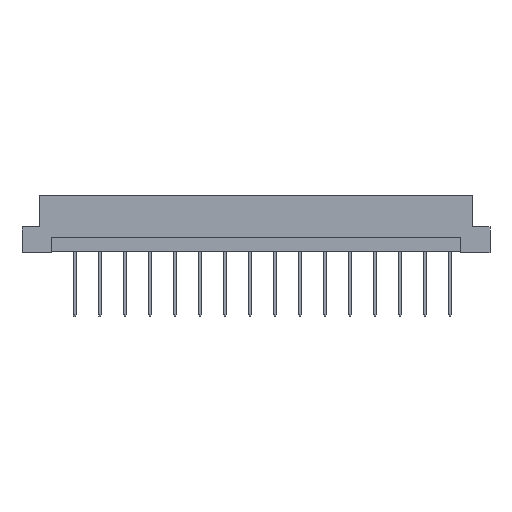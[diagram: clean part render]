
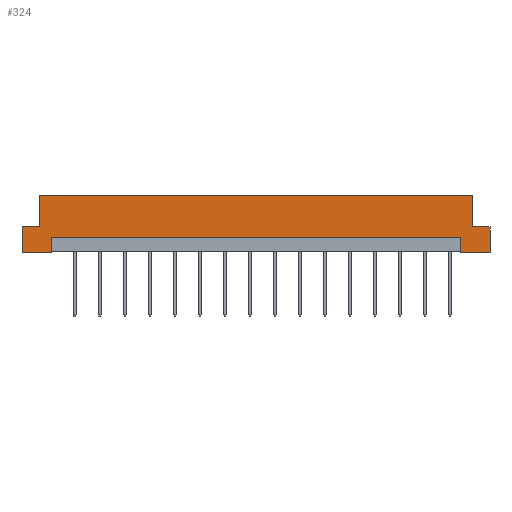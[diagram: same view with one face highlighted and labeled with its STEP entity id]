
A CAD part, front view. The second image highlights one B-rep face of the part: STEP entity #324.
In plain terms, the highlighted planar face has unit normal (0, -1, 0).
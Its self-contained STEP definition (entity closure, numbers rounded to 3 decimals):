
#177 = ORIENTED_EDGE ( 'NONE', *, *, #2732, .F. ) ;
#241 = CARTESIAN_POINT ( 'NONE',  ( 47.5, -4.3, 5.2 ) ) ;
#297 = VECTOR ( 'NONE', #2677, 1000. ) ;
#324 = ADVANCED_FACE ( 'NONE', ( #4983 ), #3222, .F. ) ;
#400 = LINE ( 'NONE', #6045, #3458 ) ;
#569 = DIRECTION ( 'NONE',  ( 1., 0., 0. ) ) ;
#707 = CARTESIAN_POINT ( 'NONE',  ( -44., -4.3, 5.2 ) ) ;
#712 = CARTESIAN_POINT ( 'NONE',  ( -44., -4.3, 5.2 ) ) ;
#802 = LINE ( 'NONE', #871, #5288 ) ;
#814 = LINE ( 'NONE', #4488, #297 ) ;
#871 = CARTESIAN_POINT ( 'NONE',  ( 47.5, -4.3, 5.2 ) ) ;
#896 = EDGE_CURVE ( 'NONE', #4671, #11580, #814, .T. ) ;
#987 = EDGE_CURVE ( 'NONE', #9827, #6473, #1780, .T. ) ;
#1007 = LINE ( 'NONE', #11076, #3887 ) ;
#1305 = LINE ( 'NONE', #8617, #1389 ) ;
#1389 = VECTOR ( 'NONE', #4064, 1000. ) ;
#1780 = LINE ( 'NONE', #9749, #8134 ) ;
#1937 = ORIENTED_EDGE ( 'NONE', *, *, #10418, .T. ) ;
#1944 = DIRECTION ( 'NONE',  ( 1., 0., 0. ) ) ;
#1977 = ORIENTED_EDGE ( 'NONE', *, *, #5237, .T. ) ;
#1996 = DIRECTION ( 'NONE',  ( 0., 0., 1. ) ) ;
#2287 = CARTESIAN_POINT ( 'NONE',  ( -41.6, -4.3, 0. ) ) ;
#2351 = LINE ( 'NONE', #6119, #2900 ) ;
#2485 = AXIS2_PLACEMENT_3D ( 'NONE', #7840, #11568, #3175 ) ;
#2677 = DIRECTION ( 'NONE',  ( 1., 0., 0. ) ) ;
#2732 = EDGE_CURVE ( 'NONE', #6263, #8411, #802, .T. ) ;
#2900 = VECTOR ( 'NONE', #5242, 1000. ) ;
#3107 = VECTOR ( 'NONE', #1996, 1000. ) ;
#3175 = DIRECTION ( 'NONE',  ( -1., 0., 0. ) ) ;
#3222 = PLANE ( 'NONE',  #2485 ) ;
#3340 = ORIENTED_EDGE ( 'NONE', *, *, #8444, .F. ) ;
#3458 = VECTOR ( 'NONE', #569, 1000. ) ;
#3590 = ORIENTED_EDGE ( 'NONE', *, *, #11292, .F. ) ;
#3747 = CARTESIAN_POINT ( 'NONE',  ( 41.6, -4.3, 0. ) ) ;
#3880 = VERTEX_POINT ( 'NONE', #8733 ) ;
#3887 = VECTOR ( 'NONE', #4741, 1000. ) ;
#3905 = CARTESIAN_POINT ( 'NONE',  ( -41.6, -4.3, 3. ) ) ;
#4009 = CARTESIAN_POINT ( 'NONE',  ( -47.5, -4.3, 5.2 ) ) ;
#4015 = LINE ( 'NONE', #6838, #11342 ) ;
#4064 = DIRECTION ( 'NONE',  ( 1., 0., 0. ) ) ;
#4167 = VERTEX_POINT ( 'NONE', #6956 ) ;
#4204 = EDGE_CURVE ( 'NONE', #6263, #11404, #1007, .T. ) ;
#4488 = CARTESIAN_POINT ( 'NONE',  ( 47.5, -4.3, 0. ) ) ;
#4540 = DIRECTION ( 'NONE',  ( 1., 0., 0. ) ) ;
#4671 = VERTEX_POINT ( 'NONE', #3747 ) ;
#4714 = LINE ( 'NONE', #10150, #7612 ) ;
#4741 = DIRECTION ( 'NONE',  ( 0., 0., 1. ) ) ;
#4983 = FACE_OUTER_BOUND ( 'NONE', #11604, .T. ) ;
#5168 = LINE ( 'NONE', #11508, #11522 ) ;
#5237 = EDGE_CURVE ( 'NONE', #9170, #6473, #4714, .T. ) ;
#5242 = DIRECTION ( 'NONE',  ( 0., 0., -1. ) ) ;
#5288 = VECTOR ( 'NONE', #4540, 1000. ) ;
#5415 = CARTESIAN_POINT ( 'NONE',  ( 47.5, -4.3, 0. ) ) ;
#5600 = LINE ( 'NONE', #5716, #3107 ) ;
#5716 = CARTESIAN_POINT ( 'NONE',  ( 41.6, -4.3, 0.2 ) ) ;
#5813 = VECTOR ( 'NONE', #10901, 1000. ) ;
#6045 = CARTESIAN_POINT ( 'NONE',  ( -41.6, -4.3, 3. ) ) ;
#6119 = CARTESIAN_POINT ( 'NONE',  ( 47.5, -4.3, 11.6 ) ) ;
#6178 = ORIENTED_EDGE ( 'NONE', *, *, #8817, .F. ) ;
#6263 = VERTEX_POINT ( 'NONE', #7809 ) ;
#6281 = DIRECTION ( 'NONE',  ( 0., 0., -1. ) ) ;
#6473 = VERTEX_POINT ( 'NONE', #2287 ) ;
#6667 = DIRECTION ( 'NONE',  ( 1., 0., 0. ) ) ;
#6725 = EDGE_CURVE ( 'NONE', #8411, #11580, #2351, .T. ) ;
#6838 = CARTESIAN_POINT ( 'NONE',  ( 47.5, -4.3, 11.6 ) ) ;
#6956 = CARTESIAN_POINT ( 'NONE',  ( -44., -4.3, 11.6 ) ) ;
#7208 = ORIENTED_EDGE ( 'NONE', *, *, #4204, .T. ) ;
#7612 = VECTOR ( 'NONE', #1944, 1000. ) ;
#7809 = CARTESIAN_POINT ( 'NONE',  ( 44., -4.3, 5.2 ) ) ;
#7816 = ORIENTED_EDGE ( 'NONE', *, *, #11731, .F. ) ;
#7840 = CARTESIAN_POINT ( 'NONE',  ( 47.5, -4.3, 11.6 ) ) ;
#7848 = ORIENTED_EDGE ( 'NONE', *, *, #6725, .F. ) ;
#7917 = CARTESIAN_POINT ( 'NONE',  ( 44., -4.3, 11.6 ) ) ;
#7979 = DIRECTION ( 'NONE',  ( 0., 0., -1. ) ) ;
#8006 = ORIENTED_EDGE ( 'NONE', *, *, #987, .F. ) ;
#8134 = VECTOR ( 'NONE', #6281, 1000. ) ;
#8411 = VERTEX_POINT ( 'NONE', #241 ) ;
#8444 = EDGE_CURVE ( 'NONE', #4671, #3880, #5600, .T. ) ;
#8547 = VERTEX_POINT ( 'NONE', #4009 ) ;
#8617 = CARTESIAN_POINT ( 'NONE',  ( -47.5, -4.3, 5.2 ) ) ;
#8733 = CARTESIAN_POINT ( 'NONE',  ( 41.6, -4.3, 3. ) ) ;
#8817 = EDGE_CURVE ( 'NONE', #11340, #4167, #9892, .T. ) ;
#9170 = VERTEX_POINT ( 'NONE', #10754 ) ;
#9248 = ORIENTED_EDGE ( 'NONE', *, *, #896, .T. ) ;
#9749 = CARTESIAN_POINT ( 'NONE',  ( -41.6, -4.3, 0.2 ) ) ;
#9827 = VERTEX_POINT ( 'NONE', #3905 ) ;
#9892 = LINE ( 'NONE', #707, #5813 ) ;
#10088 = ORIENTED_EDGE ( 'NONE', *, *, #11381, .T. ) ;
#10150 = CARTESIAN_POINT ( 'NONE',  ( 47.5, -4.3, 0. ) ) ;
#10418 = EDGE_CURVE ( 'NONE', #9827, #3880, #400, .T. ) ;
#10754 = CARTESIAN_POINT ( 'NONE',  ( -47.5, -4.3, 0. ) ) ;
#10901 = DIRECTION ( 'NONE',  ( 0., 0., 1. ) ) ;
#11076 = CARTESIAN_POINT ( 'NONE',  ( 44., -4.3, 5.2 ) ) ;
#11292 = EDGE_CURVE ( 'NONE', #4167, #11404, #4015, .T. ) ;
#11340 = VERTEX_POINT ( 'NONE', #712 ) ;
#11342 = VECTOR ( 'NONE', #6667, 1000. ) ;
#11381 = EDGE_CURVE ( 'NONE', #8547, #9170, #5168, .T. ) ;
#11404 = VERTEX_POINT ( 'NONE', #7917 ) ;
#11508 = CARTESIAN_POINT ( 'NONE',  ( -47.5, -4.3, 11.6 ) ) ;
#11522 = VECTOR ( 'NONE', #7979, 1000. ) ;
#11568 = DIRECTION ( 'NONE',  ( 0., 1., 0. ) ) ;
#11580 = VERTEX_POINT ( 'NONE', #5415 ) ;
#11604 = EDGE_LOOP ( 'NONE', ( #1937, #3340, #9248, #7848, #177, #7208, #3590, #6178, #7816, #10088, #1977, #8006 ) ) ;
#11731 = EDGE_CURVE ( 'NONE', #8547, #11340, #1305, .T. ) ;
